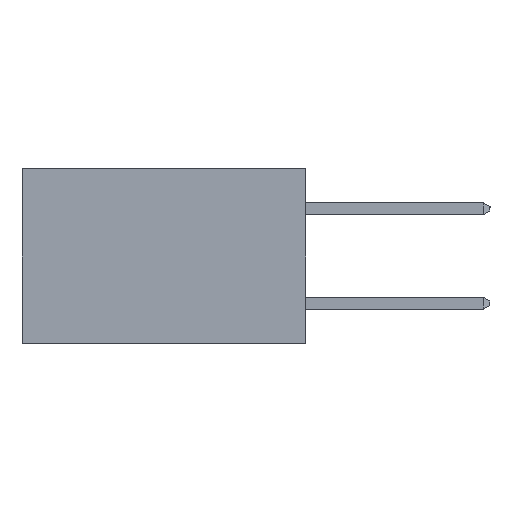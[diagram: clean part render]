
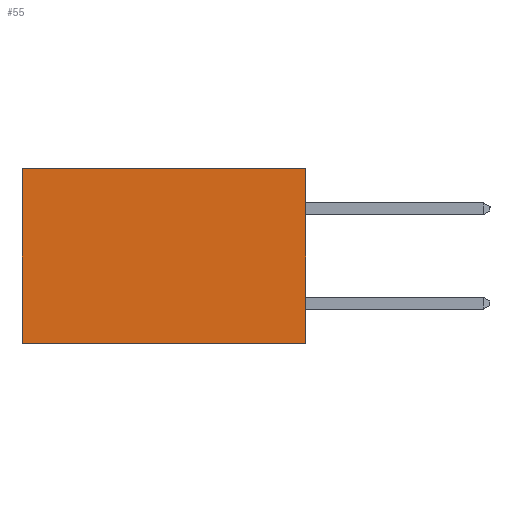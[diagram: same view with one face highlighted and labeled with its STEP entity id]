
A CAD part, left-side view. The second image highlights one B-rep face of the part: STEP entity #55.
In plain terms, the highlighted planar face has unit normal (-1, 0, 0).
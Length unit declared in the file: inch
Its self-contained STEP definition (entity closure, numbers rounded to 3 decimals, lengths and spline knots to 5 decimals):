
#55 = ADVANCED_FACE ( 'NONE', ( #16837 ), #8667, .F. ) ;
#578 = CARTESIAN_POINT ( 'NONE',  ( 0.2615, 0., 0. ) ) ;
#1534 = VECTOR ( 'NONE', #11981, 39.37008 ) ;
#1554 = EDGE_CURVE ( 'NONE', #9100, #8374, #13994, .T. ) ;
#1655 = CARTESIAN_POINT ( 'NONE',  ( 0.2615, 0., -0.37 ) ) ;
#2531 = VECTOR ( 'NONE', #15344, 39.37008 ) ;
#2978 = CARTESIAN_POINT ( 'NONE',  ( 0.2615, 0.6, -0.37 ) ) ;
#3640 = CARTESIAN_POINT ( 'NONE',  ( 0.2615, 0.6, 0. ) ) ;
#4200 = EDGE_CURVE ( 'NONE', #16737, #8374, #6794, .T. ) ;
#4228 = EDGE_LOOP ( 'NONE', ( #7095, #12139, #16130, #8931 ) ) ;
#4402 = CARTESIAN_POINT ( 'NONE',  ( 0.2615, 0., 0. ) ) ;
#4839 = AXIS2_PLACEMENT_3D ( 'NONE', #1655, #11154, #6968 ) ;
#4907 = VERTEX_POINT ( 'NONE', #578 ) ;
#5464 = CARTESIAN_POINT ( 'NONE',  ( 0.2615, 0., -0.37 ) ) ;
#5853 = EDGE_CURVE ( 'NONE', #4907, #9100, #9916, .T. ) ;
#6584 = CARTESIAN_POINT ( 'NONE',  ( 0.2615, 0., -0.37 ) ) ;
#6794 = LINE ( 'NONE', #5464, #1534 ) ;
#6968 = DIRECTION ( 'NONE',  ( 0., 0., -1. ) ) ;
#7095 = ORIENTED_EDGE ( 'NONE', *, *, #1554, .T. ) ;
#7209 = DIRECTION ( 'NONE',  ( 0., 0., -1. ) ) ;
#8134 = CARTESIAN_POINT ( 'NONE',  ( 0.2615, 0.6, -0.37 ) ) ;
#8374 = VERTEX_POINT ( 'NONE', #8134 ) ;
#8667 = PLANE ( 'NONE',  #4839 ) ;
#8931 = ORIENTED_EDGE ( 'NONE', *, *, #5853, .T. ) ;
#9100 = VERTEX_POINT ( 'NONE', #3640 ) ;
#9916 = LINE ( 'NONE', #4402, #2531 ) ;
#10057 = CARTESIAN_POINT ( 'NONE',  ( 0.2615, 0., -0.37 ) ) ;
#10781 = VECTOR ( 'NONE', #12579, 39.37008 ) ;
#11154 = DIRECTION ( 'NONE',  ( 1., 0., 0. ) ) ;
#11981 = DIRECTION ( 'NONE',  ( 0., 1., 0. ) ) ;
#12139 = ORIENTED_EDGE ( 'NONE', *, *, #4200, .F. ) ;
#12579 = DIRECTION ( 'NONE',  ( 0., 0., -1. ) ) ;
#12829 = LINE ( 'NONE', #10057, #17130 ) ;
#13994 = LINE ( 'NONE', #2978, #10781 ) ;
#15344 = DIRECTION ( 'NONE',  ( 0., 1., 0. ) ) ;
#16130 = ORIENTED_EDGE ( 'NONE', *, *, #17044, .F. ) ;
#16737 = VERTEX_POINT ( 'NONE', #6584 ) ;
#16837 = FACE_OUTER_BOUND ( 'NONE', #4228, .T. ) ;
#17044 = EDGE_CURVE ( 'NONE', #4907, #16737, #12829, .T. ) ;
#17130 = VECTOR ( 'NONE', #7209, 39.37008 ) ;
